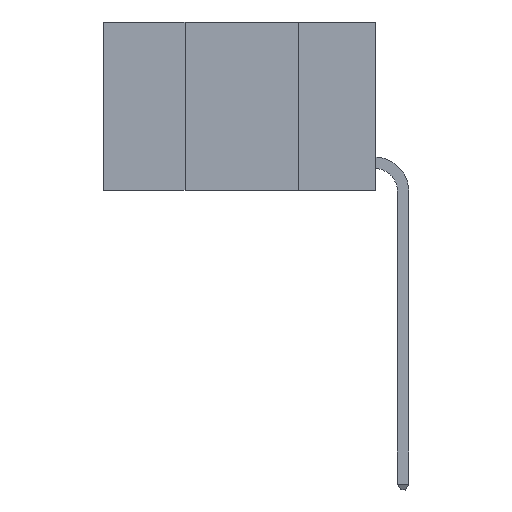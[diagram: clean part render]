
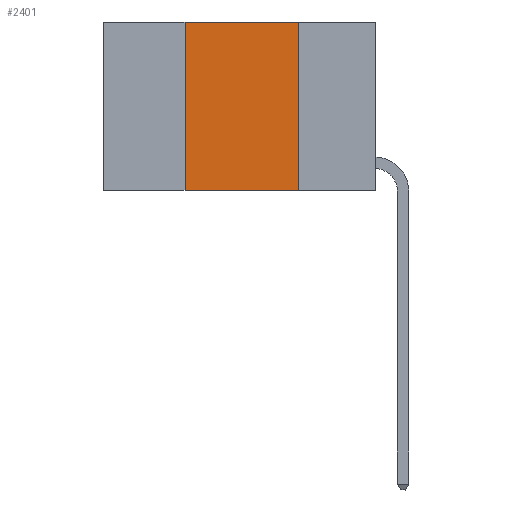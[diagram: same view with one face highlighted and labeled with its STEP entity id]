
A CAD part, left-side view. The second image highlights one B-rep face of the part: STEP entity #2401.
In plain terms, the highlighted planar face has unit normal (-1, 0, 0).
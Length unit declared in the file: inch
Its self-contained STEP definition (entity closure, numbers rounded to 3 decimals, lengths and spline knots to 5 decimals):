
#91 = ORIENTED_EDGE ( 'NONE', *, *, #2118, .T. ) ;
#373 = AXIS2_PLACEMENT_3D ( 'NONE', #4470, #4410, #4391 ) ;
#796 = VECTOR ( 'NONE', #1675, 39.37008 ) ;
#904 = VECTOR ( 'NONE', #6804, 39.37008 ) ;
#944 = LINE ( 'NONE', #1913, #7476 ) ;
#980 = CARTESIAN_POINT ( 'NONE',  ( 0., 0.17, 0. ) ) ;
#1029 = LINE ( 'NONE', #980, #796 ) ;
#1123 = CARTESIAN_POINT ( 'NONE',  ( 0., 0.17, 0. ) ) ;
#1250 = VERTEX_POINT ( 'NONE', #3652 ) ;
#1287 = EDGE_LOOP ( 'NONE', ( #2913, #6678, #3564, #91 ) ) ;
#1675 = DIRECTION ( 'NONE',  ( 0., 0., -1. ) ) ;
#1719 = CARTESIAN_POINT ( 'NONE',  ( 0., 0.6, 0. ) ) ;
#1913 = CARTESIAN_POINT ( 'NONE',  ( 0., 0.42, 0. ) ) ;
#1942 = DIRECTION ( 'NONE',  ( 0., 0., 1. ) ) ;
#2118 = EDGE_CURVE ( 'NONE', #3046, #1250, #4686, .T. ) ;
#2401 = ADVANCED_FACE ( 'NONE', ( #7223 ), #4544, .F. ) ;
#2552 = EDGE_CURVE ( 'NONE', #3046, #6703, #944, .T. ) ;
#2793 = CARTESIAN_POINT ( 'NONE',  ( 0., 0.42, 0. ) ) ;
#2913 = ORIENTED_EDGE ( 'NONE', *, *, #4340, .F. ) ;
#3046 = VERTEX_POINT ( 'NONE', #7771 ) ;
#3564 = ORIENTED_EDGE ( 'NONE', *, *, #2552, .F. ) ;
#3652 = CARTESIAN_POINT ( 'NONE',  ( 0., 0.17, -0.37 ) ) ;
#4340 = EDGE_CURVE ( 'NONE', #5757, #1250, #1029, .T. ) ;
#4391 = DIRECTION ( 'NONE',  ( 0., 0., -1. ) ) ;
#4410 = DIRECTION ( 'NONE',  ( 1., 0., 0. ) ) ;
#4470 = CARTESIAN_POINT ( 'NONE',  ( 0., 0.6, 0. ) ) ;
#4544 = PLANE ( 'NONE',  #373 ) ;
#4686 = LINE ( 'NONE', #8008, #7662 ) ;
#4983 = EDGE_CURVE ( 'NONE', #6703, #5757, #7630, .T. ) ;
#5757 = VERTEX_POINT ( 'NONE', #1123 ) ;
#6678 = ORIENTED_EDGE ( 'NONE', *, *, #4983, .F. ) ;
#6703 = VERTEX_POINT ( 'NONE', #2793 ) ;
#6804 = DIRECTION ( 'NONE',  ( 0., -1., 0. ) ) ;
#7223 = FACE_OUTER_BOUND ( 'NONE', #1287, .T. ) ;
#7476 = VECTOR ( 'NONE', #1942, 39.37008 ) ;
#7630 = LINE ( 'NONE', #1719, #904 ) ;
#7662 = VECTOR ( 'NONE', #7825, 39.37008 ) ;
#7771 = CARTESIAN_POINT ( 'NONE',  ( 0., 0.42, -0.37 ) ) ;
#7825 = DIRECTION ( 'NONE',  ( 0., -1., 0. ) ) ;
#8008 = CARTESIAN_POINT ( 'NONE',  ( 0., 0.6, -0.37 ) ) ;
